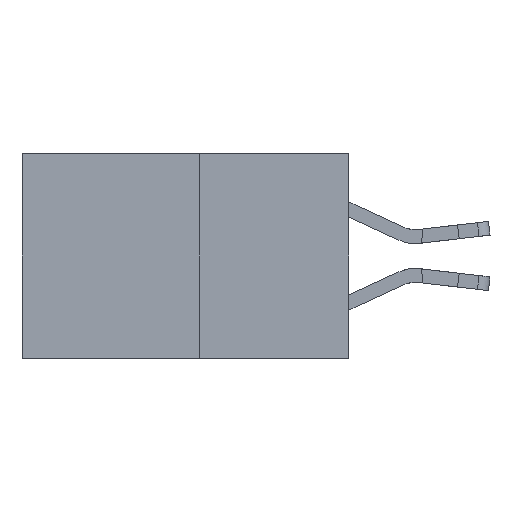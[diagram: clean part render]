
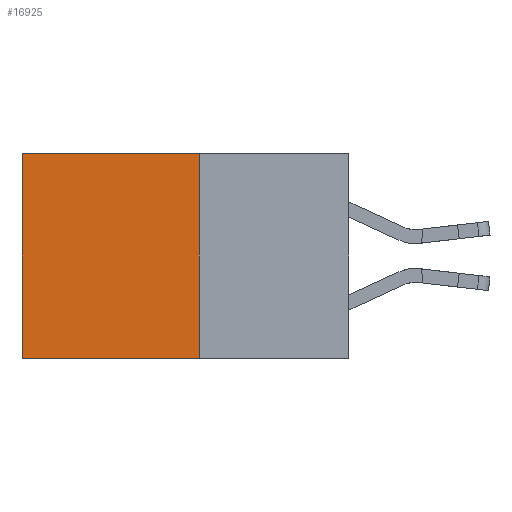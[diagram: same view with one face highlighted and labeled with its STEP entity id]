
A CAD part, left-side view. The second image highlights one B-rep face of the part: STEP entity #16925.
In plain terms, the highlighted planar face has unit normal (-1, 0, 0).
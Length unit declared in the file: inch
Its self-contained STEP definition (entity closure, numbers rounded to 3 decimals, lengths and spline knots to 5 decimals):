
#571 = VERTEX_POINT ( 'NONE', #10010 ) ;
#573 = EDGE_CURVE ( 'NONE', #571, #11283, #10125, .T. ) ;
#894 = CARTESIAN_POINT ( 'NONE',  ( 0.277, 0.59, 0. ) ) ;
#1718 = EDGE_CURVE ( 'NONE', #11405, #9659, #9266, .T. ) ;
#2880 = ORIENTED_EDGE ( 'NONE', *, *, #1718, .T. ) ;
#3035 = VECTOR ( 'NONE', #12707, 39.37008 ) ;
#3547 = ORIENTED_EDGE ( 'NONE', *, *, #4724, .F. ) ;
#3998 = CARTESIAN_POINT ( 'NONE',  ( 0.277, 0.59, -0.37 ) ) ;
#4084 = CARTESIAN_POINT ( 'NONE',  ( 0.277, 0.27, -0.37 ) ) ;
#4544 = EDGE_LOOP ( 'NONE', ( #2880, #3547, #8795, #9212 ) ) ;
#4724 = EDGE_CURVE ( 'NONE', #11283, #9659, #10707, .T. ) ;
#4937 = CARTESIAN_POINT ( 'NONE',  ( 0.277, 0.59, -0.37 ) ) ;
#5214 = EDGE_CURVE ( 'NONE', #571, #11405, #16730, .T. ) ;
#5409 = DIRECTION ( 'NONE',  ( 0., 0., -1. ) ) ;
#5481 = PLANE ( 'NONE',  #7337 ) ;
#5815 = CARTESIAN_POINT ( 'NONE',  ( 0.277, 0.27, -0.37 ) ) ;
#6326 = VECTOR ( 'NONE', #14303, 39.37008 ) ;
#6621 = FACE_OUTER_BOUND ( 'NONE', #4544, .T. ) ;
#6761 = VECTOR ( 'NONE', #11875, 39.37008 ) ;
#7337 = AXIS2_PLACEMENT_3D ( 'NONE', #4084, #13323, #5409 ) ;
#8274 = CARTESIAN_POINT ( 'NONE',  ( 0.277, 0.27, -0.37 ) ) ;
#8350 = CARTESIAN_POINT ( 'NONE',  ( 0.277, 0.27, -0.37 ) ) ;
#8795 = ORIENTED_EDGE ( 'NONE', *, *, #573, .F. ) ;
#9212 = ORIENTED_EDGE ( 'NONE', *, *, #5214, .T. ) ;
#9266 = LINE ( 'NONE', #4937, #16981 ) ;
#9659 = VERTEX_POINT ( 'NONE', #3998 ) ;
#10010 = CARTESIAN_POINT ( 'NONE',  ( 0.277, 0.27, 0. ) ) ;
#10125 = LINE ( 'NONE', #8274, #3035 ) ;
#10707 = LINE ( 'NONE', #8350, #6761 ) ;
#11283 = VERTEX_POINT ( 'NONE', #5815 ) ;
#11405 = VERTEX_POINT ( 'NONE', #894 ) ;
#11875 = DIRECTION ( 'NONE',  ( 0., 1., 0. ) ) ;
#12707 = DIRECTION ( 'NONE',  ( 0., 0., -1. ) ) ;
#13323 = DIRECTION ( 'NONE',  ( 1., 0., 0. ) ) ;
#14303 = DIRECTION ( 'NONE',  ( 0., 1., 0. ) ) ;
#14654 = CARTESIAN_POINT ( 'NONE',  ( 0.277, 0.27, 0. ) ) ;
#16730 = LINE ( 'NONE', #14654, #6326 ) ;
#16861 = DIRECTION ( 'NONE',  ( 0., 0., -1. ) ) ;
#16925 = ADVANCED_FACE ( 'NONE', ( #6621 ), #5481, .F. ) ;
#16981 = VECTOR ( 'NONE', #16861, 39.37008 ) ;
